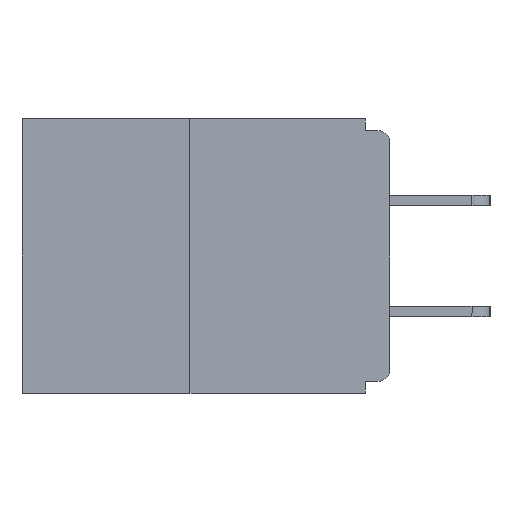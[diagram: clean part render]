
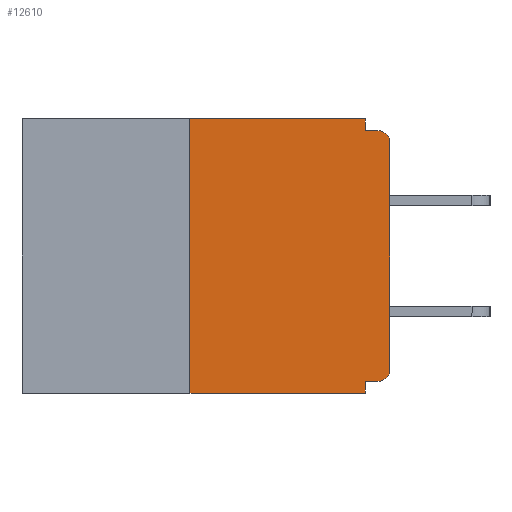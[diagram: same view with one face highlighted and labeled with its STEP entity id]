
A CAD part, left-side view. The second image highlights one B-rep face of the part: STEP entity #12610.
In plain terms, the highlighted planar face has unit normal (-1, 0, 0).
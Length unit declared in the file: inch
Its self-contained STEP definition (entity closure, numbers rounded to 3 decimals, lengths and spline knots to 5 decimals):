
#146 = ORIENTED_EDGE ( 'NONE', *, *, #4955, .F. ) ;
#409 = LINE ( 'NONE', #11959, #23572 ) ;
#724 = CARTESIAN_POINT ( 'NONE',  ( 0., 0.015, -0.313 ) ) ;
#1333 = CIRCLE ( 'NONE', #2713, 0.015 ) ;
#1912 = CARTESIAN_POINT ( 'NONE',  ( 0., 0.031, -0.015 ) ) ;
#2369 = EDGE_CURVE ( 'NONE', #6351, #16302, #4615, .T. ) ;
#2559 = LINE ( 'NONE', #23197, #19365 ) ;
#2713 = AXIS2_PLACEMENT_3D ( 'NONE', #724, #7551, #16437 ) ;
#2723 = EDGE_CURVE ( 'NONE', #25280, #18043, #23509, .T. ) ;
#3290 = EDGE_CURVE ( 'NONE', #6764, #23363, #13023, .T. ) ;
#3436 = AXIS2_PLACEMENT_3D ( 'NONE', #15369, #26576, #23203 ) ;
#3697 = AXIS2_PLACEMENT_3D ( 'NONE', #27079, #26891, #8961 ) ;
#3923 = ORIENTED_EDGE ( 'NONE', *, *, #3290, .T. ) ;
#4615 = LINE ( 'NONE', #9112, #28760 ) ;
#4939 = CIRCLE ( 'NONE', #3436, 0.015 ) ;
#4955 = EDGE_CURVE ( 'NONE', #24334, #6351, #16097, .T. ) ;
#5085 = CARTESIAN_POINT ( 'NONE',  ( 0., 0.031, 0. ) ) ;
#6351 = VERTEX_POINT ( 'NONE', #1912 ) ;
#6764 = VERTEX_POINT ( 'NONE', #24683 ) ;
#6952 = FACE_OUTER_BOUND ( 'NONE', #9353, .T. ) ;
#7545 = VECTOR ( 'NONE', #13737, 39.37008 ) ;
#7551 = DIRECTION ( 'NONE',  ( -1., 0., 0. ) ) ;
#7726 = CARTESIAN_POINT ( 'NONE',  ( 0., 0.015, -0.328 ) ) ;
#8325 = VECTOR ( 'NONE', #16509, 39.37008 ) ;
#8581 = VECTOR ( 'NONE', #14591, 39.37008 ) ;
#8804 = VECTOR ( 'NONE', #12770, 39.37008 ) ;
#8961 = DIRECTION ( 'NONE',  ( 0., 0., -1. ) ) ;
#9112 = CARTESIAN_POINT ( 'NONE',  ( 0., 0., -0.015 ) ) ;
#9353 = EDGE_LOOP ( 'NONE', ( #10660, #10265, #15122, #28763, #21797, #16014, #3923, #28351, #22838, #146 ) ) ;
#9499 = DIRECTION ( 'NONE',  ( 0., -1., 0. ) ) ;
#10265 = ORIENTED_EDGE ( 'NONE', *, *, #2723, .F. ) ;
#10660 = ORIENTED_EDGE ( 'NONE', *, *, #27968, .F. ) ;
#11959 = CARTESIAN_POINT ( 'NONE',  ( 0., 0.46, -0.343 ) ) ;
#12459 = LINE ( 'NONE', #27464, #7545 ) ;
#12610 = ADVANCED_FACE ( 'NONE', ( #6952 ), #18041, .F. ) ;
#12770 = DIRECTION ( 'NONE',  ( 0., 0., 1. ) ) ;
#13023 = LINE ( 'NONE', #13946, #8804 ) ;
#13737 = DIRECTION ( 'NONE',  ( 0., 0., -1. ) ) ;
#13946 = CARTESIAN_POINT ( 'NONE',  ( 0., 0., 0. ) ) ;
#14591 = DIRECTION ( 'NONE',  ( 0., 0., 1. ) ) ;
#14973 = LINE ( 'NONE', #18470, #8325 ) ;
#15122 = ORIENTED_EDGE ( 'NONE', *, *, #27354, .T. ) ;
#15369 = CARTESIAN_POINT ( 'NONE',  ( 0., 0.015, -0.03 ) ) ;
#15606 = EDGE_CURVE ( 'NONE', #18401, #24460, #14973, .T. ) ;
#16014 = ORIENTED_EDGE ( 'NONE', *, *, #23168, .T. ) ;
#16097 = LINE ( 'NONE', #5085, #27979 ) ;
#16302 = VERTEX_POINT ( 'NONE', #24376 ) ;
#16437 = DIRECTION ( 'NONE',  ( 0., 0., -1. ) ) ;
#16509 = DIRECTION ( 'NONE',  ( 0., 1., 0. ) ) ;
#16972 = VERTEX_POINT ( 'NONE', #19657 ) ;
#18041 = PLANE ( 'NONE',  #3697 ) ;
#18043 = VERTEX_POINT ( 'NONE', #24375 ) ;
#18315 = EDGE_CURVE ( 'NONE', #23363, #16302, #4939, .T. ) ;
#18401 = VERTEX_POINT ( 'NONE', #7726 ) ;
#18470 = CARTESIAN_POINT ( 'NONE',  ( 0., 0., -0.328 ) ) ;
#19365 = VECTOR ( 'NONE', #25064, 39.37008 ) ;
#19657 = CARTESIAN_POINT ( 'NONE',  ( 0., 0.031, -0.343 ) ) ;
#21386 = CARTESIAN_POINT ( 'NONE',  ( 0., 0.25, -0.343 ) ) ;
#21797 = ORIENTED_EDGE ( 'NONE', *, *, #15606, .F. ) ;
#22838 = ORIENTED_EDGE ( 'NONE', *, *, #2369, .F. ) ;
#23060 = DIRECTION ( 'NONE',  ( 0., -1., 0. ) ) ;
#23142 = CARTESIAN_POINT ( 'NONE',  ( 0., 0.031, 0. ) ) ;
#23168 = EDGE_CURVE ( 'NONE', #18401, #6764, #1333, .T. ) ;
#23197 = CARTESIAN_POINT ( 'NONE',  ( 0., 0.46, 0. ) ) ;
#23203 = DIRECTION ( 'NONE',  ( 0., 0., -1. ) ) ;
#23363 = VERTEX_POINT ( 'NONE', #28419 ) ;
#23509 = LINE ( 'NONE', #27951, #8581 ) ;
#23572 = VECTOR ( 'NONE', #23060, 39.37008 ) ;
#24334 = VERTEX_POINT ( 'NONE', #23142 ) ;
#24375 = CARTESIAN_POINT ( 'NONE',  ( 0., 0.25, 0. ) ) ;
#24376 = CARTESIAN_POINT ( 'NONE',  ( 0., 0.015, -0.015 ) ) ;
#24460 = VERTEX_POINT ( 'NONE', #25870 ) ;
#24683 = CARTESIAN_POINT ( 'NONE',  ( 0., 0., -0.313 ) ) ;
#25064 = DIRECTION ( 'NONE',  ( 0., -1., 0. ) ) ;
#25280 = VERTEX_POINT ( 'NONE', #21386 ) ;
#25523 = DIRECTION ( 'NONE',  ( 0., 0., -1. ) ) ;
#25870 = CARTESIAN_POINT ( 'NONE',  ( 0., 0.031, -0.328 ) ) ;
#26576 = DIRECTION ( 'NONE',  ( -1., 0., 0. ) ) ;
#26623 = EDGE_CURVE ( 'NONE', #24460, #16972, #12459, .T. ) ;
#26891 = DIRECTION ( 'NONE',  ( 1., 0., 0. ) ) ;
#27079 = CARTESIAN_POINT ( 'NONE',  ( 0., 0.46, 0. ) ) ;
#27354 = EDGE_CURVE ( 'NONE', #25280, #16972, #409, .T. ) ;
#27464 = CARTESIAN_POINT ( 'NONE',  ( 0., 0.031, -0.343 ) ) ;
#27951 = CARTESIAN_POINT ( 'NONE',  ( 0., 0.25, 0. ) ) ;
#27968 = EDGE_CURVE ( 'NONE', #18043, #24334, #2559, .T. ) ;
#27979 = VECTOR ( 'NONE', #25523, 39.37008 ) ;
#28351 = ORIENTED_EDGE ( 'NONE', *, *, #18315, .T. ) ;
#28419 = CARTESIAN_POINT ( 'NONE',  ( 0., 0., -0.03 ) ) ;
#28760 = VECTOR ( 'NONE', #9499, 39.37008 ) ;
#28763 = ORIENTED_EDGE ( 'NONE', *, *, #26623, .F. ) ;
